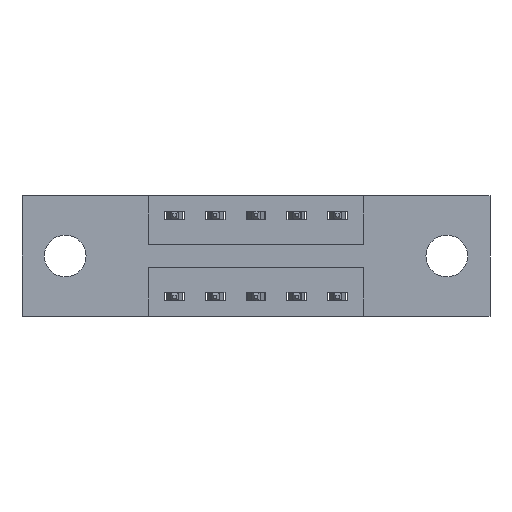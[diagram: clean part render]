
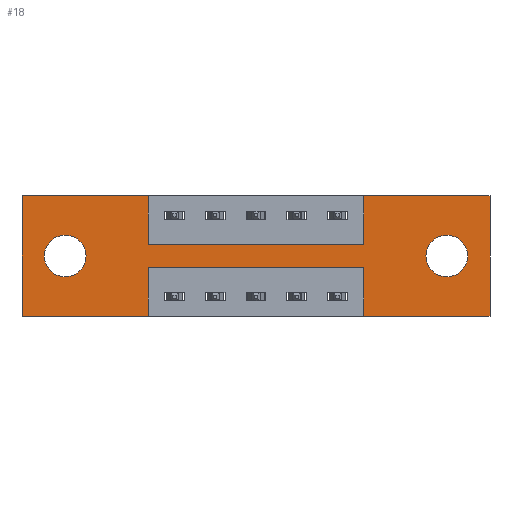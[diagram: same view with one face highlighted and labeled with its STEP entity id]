
A CAD part, front view. The second image highlights one B-rep face of the part: STEP entity #18.
In plain terms, the highlighted planar face has unit normal (0, -1, 0).
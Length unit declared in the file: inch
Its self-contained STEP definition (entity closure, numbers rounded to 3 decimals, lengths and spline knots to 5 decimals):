
#18 = ADVANCED_FACE ( 'NONE', ( #2169, #299, #6971 ), #4537, .T. ) ;
#38 = CARTESIAN_POINT ( 'NONE',  ( 0.3875, 0., -0.22 ) ) ;
#115 = EDGE_CURVE ( 'NONE', #6219, #6996, #1505, .T. ) ;
#250 = DIRECTION ( 'NONE',  ( 1., 0., 0. ) ) ;
#252 = DIRECTION ( 'NONE',  ( 0., -1., 0. ) ) ;
#299 = FACE_BOUND ( 'NONE', #2958, .T. ) ;
#334 = CIRCLE ( 'NONE', #4594, 0.064 ) ;
#351 = ORIENTED_EDGE ( 'NONE', *, *, #4973, .T. ) ;
#384 = CARTESIAN_POINT ( 'NONE',  ( 1.3025, 0., -0.249 ) ) ;
#387 = AXIS2_PLACEMENT_3D ( 'NONE', #4893, #252, #7684 ) ;
#392 = EDGE_LOOP ( 'NONE', ( #6250, #6854, #3336, #8091, #6364, #6487, #7795, #5544, #3257, #6813, #1019, #6450 ) ) ;
#396 = DIRECTION ( 'NONE',  ( 0., 1., 0. ) ) ;
#400 = ORIENTED_EDGE ( 'NONE', *, *, #3942, .T. ) ;
#423 = CARTESIAN_POINT ( 'NONE',  ( 1.3025, 0., -0.121 ) ) ;
#615 = LINE ( 'NONE', #7558, #7054 ) ;
#641 = DIRECTION ( 'NONE',  ( 0., 0., -1. ) ) ;
#650 = VECTOR ( 'NONE', #4246, 39.37008 ) ;
#667 = ORIENTED_EDGE ( 'NONE', *, *, #3832, .T. ) ;
#758 = CARTESIAN_POINT ( 'NONE',  ( 0.3875, 0., -0.22 ) ) ;
#769 = EDGE_LOOP ( 'NONE', ( #667, #400 ) ) ;
#966 = CARTESIAN_POINT ( 'NONE',  ( 0.1325, 0., -0.185 ) ) ;
#1019 = ORIENTED_EDGE ( 'NONE', *, *, #6344, .F. ) ;
#1031 = LINE ( 'NONE', #3121, #6136 ) ;
#1103 = CARTESIAN_POINT ( 'NONE',  ( 0., 0., -0.37 ) ) ;
#1234 = VERTEX_POINT ( 'NONE', #8128 ) ;
#1310 = DIRECTION ( 'NONE',  ( -1., 0., 0. ) ) ;
#1400 = CARTESIAN_POINT ( 'NONE',  ( 0., 0., 0. ) ) ;
#1505 = LINE ( 'NONE', #5769, #8018 ) ;
#1645 = EDGE_CURVE ( 'NONE', #5976, #2461, #4106, .T. ) ;
#1653 = CARTESIAN_POINT ( 'NONE',  ( 0.3875, 0., -0.37 ) ) ;
#1856 = VERTEX_POINT ( 'NONE', #423 ) ;
#1895 = VERTEX_POINT ( 'NONE', #38 ) ;
#1973 = EDGE_CURVE ( 'NONE', #2003, #2299, #6338, .T. ) ;
#2003 = VERTEX_POINT ( 'NONE', #4136 ) ;
#2104 = DIRECTION ( 'NONE',  ( 1., 0., 0. ) ) ;
#2132 = CARTESIAN_POINT ( 'NONE',  ( 1.3025, 0., -0.185 ) ) ;
#2169 = FACE_BOUND ( 'NONE', #769, .T. ) ;
#2267 = CARTESIAN_POINT ( 'NONE',  ( 0.3875, 0., 0. ) ) ;
#2299 = VERTEX_POINT ( 'NONE', #3126 ) ;
#2314 = CARTESIAN_POINT ( 'NONE',  ( 1.0475, 0., -0.37 ) ) ;
#2402 = CARTESIAN_POINT ( 'NONE',  ( 1.0475, 0., -0.22 ) ) ;
#2407 = VERTEX_POINT ( 'NONE', #6300 ) ;
#2461 = VERTEX_POINT ( 'NONE', #7594 ) ;
#2538 = DIRECTION ( 'NONE',  ( -1., 0., 0. ) ) ;
#2562 = DIRECTION ( 'NONE',  ( 0., 1., 0. ) ) ;
#2644 = EDGE_CURVE ( 'NONE', #4196, #1234, #4183, .T. ) ;
#2777 = DIRECTION ( 'NONE',  ( 0., 0., -1. ) ) ;
#2789 = EDGE_CURVE ( 'NONE', #4232, #1895, #3410, .T. ) ;
#2880 = CARTESIAN_POINT ( 'NONE',  ( 0.1325, 0., -0.249 ) ) ;
#2892 = CIRCLE ( 'NONE', #5417, 0.064 ) ;
#2958 = EDGE_LOOP ( 'NONE', ( #351, #6274 ) ) ;
#2973 = EDGE_CURVE ( 'NONE', #2407, #3174, #5337, .T. ) ;
#2980 = DIRECTION ( 'NONE',  ( 0., 0., 1. ) ) ;
#3025 = VECTOR ( 'NONE', #1310, 39.37008 ) ;
#3087 = CARTESIAN_POINT ( 'NONE',  ( 1.435, 0., -0.37 ) ) ;
#3121 = CARTESIAN_POINT ( 'NONE',  ( 1.435, 0., 0. ) ) ;
#3126 = CARTESIAN_POINT ( 'NONE',  ( 0., 0., -0.37 ) ) ;
#3133 = VECTOR ( 'NONE', #6202, 39.37008 ) ;
#3174 = VERTEX_POINT ( 'NONE', #3194 ) ;
#3194 = CARTESIAN_POINT ( 'NONE',  ( 1.0475, 0., -0.15 ) ) ;
#3229 = VECTOR ( 'NONE', #6007, 39.37008 ) ;
#3257 = ORIENTED_EDGE ( 'NONE', *, *, #6669, .F. ) ;
#3336 = ORIENTED_EDGE ( 'NONE', *, *, #4139, .F. ) ;
#3410 = LINE ( 'NONE', #758, #4880 ) ;
#3691 = CARTESIAN_POINT ( 'NONE',  ( 1.0475, 0., 0. ) ) ;
#3832 = EDGE_CURVE ( 'NONE', #1856, #5677, #334, .T. ) ;
#3920 = EDGE_CURVE ( 'NONE', #5046, #4394, #7849, .T. ) ;
#3930 = CIRCLE ( 'NONE', #7471, 0.064 ) ;
#3942 = EDGE_CURVE ( 'NONE', #5677, #1856, #2892, .T. ) ;
#4106 = CIRCLE ( 'NONE', #6679, 0.064 ) ;
#4136 = CARTESIAN_POINT ( 'NONE',  ( 0.3875, 0., -0.37 ) ) ;
#4139 = EDGE_CURVE ( 'NONE', #6996, #4232, #6705, .T. ) ;
#4141 = LINE ( 'NONE', #1653, #650 ) ;
#4183 = LINE ( 'NONE', #5247, #7505 ) ;
#4196 = VERTEX_POINT ( 'NONE', #7962 ) ;
#4220 = DIRECTION ( 'NONE',  ( 1., 0., 0. ) ) ;
#4232 = VERTEX_POINT ( 'NONE', #2402 ) ;
#4246 = DIRECTION ( 'NONE',  ( 0., 0., -1. ) ) ;
#4362 = CARTESIAN_POINT ( 'NONE',  ( 0.1325, 0., -0.185 ) ) ;
#4394 = VERTEX_POINT ( 'NONE', #7562 ) ;
#4537 = PLANE ( 'NONE',  #387 ) ;
#4551 = DIRECTION ( 'NONE',  ( 0., 1., 0. ) ) ;
#4594 = AXIS2_PLACEMENT_3D ( 'NONE', #8241, #4551, #641 ) ;
#4801 = LINE ( 'NONE', #3691, #3133 ) ;
#4867 = EDGE_CURVE ( 'NONE', #1895, #2003, #4141, .T. ) ;
#4880 = VECTOR ( 'NONE', #5902, 39.37008 ) ;
#4893 = CARTESIAN_POINT ( 'NONE',  ( 0., 0., -0.37 ) ) ;
#4973 = EDGE_CURVE ( 'NONE', #2461, #5976, #3930, .T. ) ;
#4989 = DIRECTION ( 'NONE',  ( 0., 0., 1. ) ) ;
#5046 = VERTEX_POINT ( 'NONE', #5650 ) ;
#5247 = CARTESIAN_POINT ( 'NONE',  ( 0., 0., 0. ) ) ;
#5337 = LINE ( 'NONE', #5464, #8230 ) ;
#5417 = AXIS2_PLACEMENT_3D ( 'NONE', #2132, #6501, #2777 ) ;
#5464 = CARTESIAN_POINT ( 'NONE',  ( 0.3875, 0., -0.15 ) ) ;
#5544 = ORIENTED_EDGE ( 'NONE', *, *, #2973, .F. ) ;
#5627 = DIRECTION ( 'NONE',  ( 0., 0., -1. ) ) ;
#5650 = CARTESIAN_POINT ( 'NONE',  ( 1.0475, 0., 0. ) ) ;
#5677 = VERTEX_POINT ( 'NONE', #384 ) ;
#5769 = CARTESIAN_POINT ( 'NONE',  ( 0., 0., -0.37 ) ) ;
#5902 = DIRECTION ( 'NONE',  ( -1., 0., 0. ) ) ;
#5976 = VERTEX_POINT ( 'NONE', #2880 ) ;
#6007 = DIRECTION ( 'NONE',  ( 0., 0., -1. ) ) ;
#6136 = VECTOR ( 'NONE', #5627, 39.37008 ) ;
#6202 = DIRECTION ( 'NONE',  ( 0., 0., 1. ) ) ;
#6218 = VECTOR ( 'NONE', #2104, 39.37008 ) ;
#6219 = VERTEX_POINT ( 'NONE', #3087 ) ;
#6250 = ORIENTED_EDGE ( 'NONE', *, *, #4867, .F. ) ;
#6274 = ORIENTED_EDGE ( 'NONE', *, *, #1645, .T. ) ;
#6300 = CARTESIAN_POINT ( 'NONE',  ( 0.3875, 0., -0.15 ) ) ;
#6332 = DIRECTION ( 'NONE',  ( 0., 0., 1. ) ) ;
#6338 = LINE ( 'NONE', #1103, #3025 ) ;
#6344 = EDGE_CURVE ( 'NONE', #2299, #4196, #615, .T. ) ;
#6347 = LINE ( 'NONE', #2267, #3229 ) ;
#6364 = ORIENTED_EDGE ( 'NONE', *, *, #8008, .F. ) ;
#6450 = ORIENTED_EDGE ( 'NONE', *, *, #1973, .F. ) ;
#6487 = ORIENTED_EDGE ( 'NONE', *, *, #3920, .F. ) ;
#6501 = DIRECTION ( 'NONE',  ( 0., 1., 0. ) ) ;
#6669 = EDGE_CURVE ( 'NONE', #1234, #2407, #6347, .T. ) ;
#6679 = AXIS2_PLACEMENT_3D ( 'NONE', #966, #2562, #2980 ) ;
#6705 = LINE ( 'NONE', #2314, #8134 ) ;
#6813 = ORIENTED_EDGE ( 'NONE', *, *, #2644, .F. ) ;
#6839 = EDGE_CURVE ( 'NONE', #3174, #5046, #4801, .T. ) ;
#6854 = ORIENTED_EDGE ( 'NONE', *, *, #2789, .F. ) ;
#6971 = FACE_OUTER_BOUND ( 'NONE', #392, .T. ) ;
#6996 = VERTEX_POINT ( 'NONE', #8174 ) ;
#7054 = VECTOR ( 'NONE', #6332, 39.37008 ) ;
#7312 = DIRECTION ( 'NONE',  ( 0., 0., 1. ) ) ;
#7471 = AXIS2_PLACEMENT_3D ( 'NONE', #4362, #396, #4989 ) ;
#7505 = VECTOR ( 'NONE', #4220, 39.37008 ) ;
#7558 = CARTESIAN_POINT ( 'NONE',  ( 0., 0., 0. ) ) ;
#7562 = CARTESIAN_POINT ( 'NONE',  ( 1.435, 0., 0. ) ) ;
#7594 = CARTESIAN_POINT ( 'NONE',  ( 0.1325, 0., -0.121 ) ) ;
#7684 = DIRECTION ( 'NONE',  ( 0., 0., -1. ) ) ;
#7795 = ORIENTED_EDGE ( 'NONE', *, *, #6839, .F. ) ;
#7849 = LINE ( 'NONE', #1400, #6218 ) ;
#7962 = CARTESIAN_POINT ( 'NONE',  ( 0., 0., 0. ) ) ;
#8008 = EDGE_CURVE ( 'NONE', #4394, #6219, #1031, .T. ) ;
#8018 = VECTOR ( 'NONE', #2538, 39.37008 ) ;
#8091 = ORIENTED_EDGE ( 'NONE', *, *, #115, .F. ) ;
#8128 = CARTESIAN_POINT ( 'NONE',  ( 0.3875, 0., 0. ) ) ;
#8134 = VECTOR ( 'NONE', #7312, 39.37008 ) ;
#8174 = CARTESIAN_POINT ( 'NONE',  ( 1.0475, 0., -0.37 ) ) ;
#8230 = VECTOR ( 'NONE', #250, 39.37008 ) ;
#8241 = CARTESIAN_POINT ( 'NONE',  ( 1.3025, 0., -0.185 ) ) ;
